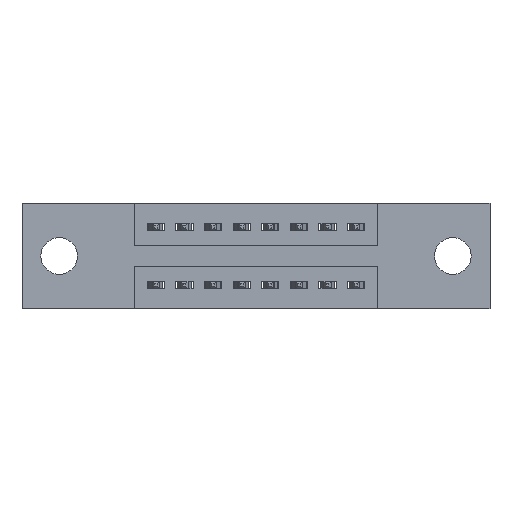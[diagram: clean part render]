
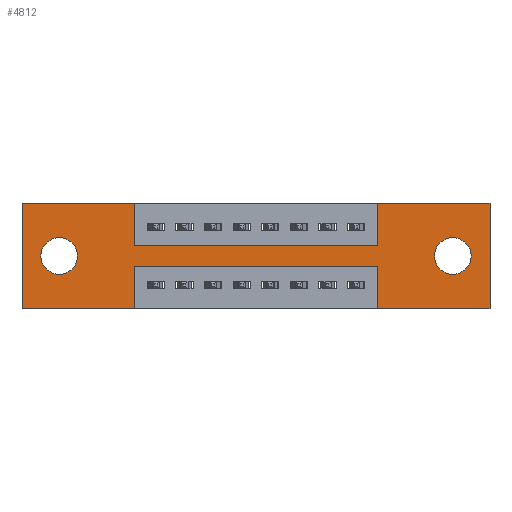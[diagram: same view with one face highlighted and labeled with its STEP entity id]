
A CAD part, front view. The second image highlights one B-rep face of the part: STEP entity #4812.
In plain terms, the highlighted planar face has unit normal (0, -1, 0).
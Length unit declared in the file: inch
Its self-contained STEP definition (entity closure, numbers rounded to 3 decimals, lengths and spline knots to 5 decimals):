
#135 = CARTESIAN_POINT ( 'NONE',  ( 0.13, 0., -0.121 ) ) ;
#247 = EDGE_CURVE ( 'NONE', #3289, #3170, #8852, .T. ) ;
#437 = LINE ( 'NONE', #5428, #8921 ) ;
#713 = VECTOR ( 'NONE', #811, 39.37008 ) ;
#737 = LINE ( 'NONE', #5722, #1028 ) ;
#811 = DIRECTION ( 'NONE',  ( 1., 0., 0. ) ) ;
#824 = CARTESIAN_POINT ( 'NONE',  ( 1.505, 0., -0.185 ) ) ;
#1003 = DIRECTION ( 'NONE',  ( 0., 0., -1. ) ) ;
#1018 = AXIS2_PLACEMENT_3D ( 'NONE', #5885, #7591, #2470 ) ;
#1028 = VECTOR ( 'NONE', #5741, 39.37008 ) ;
#1052 = LINE ( 'NONE', #7585, #7589 ) ;
#1186 = CARTESIAN_POINT ( 'NONE',  ( 1.2425, 0., -0.37 ) ) ;
#1396 = CARTESIAN_POINT ( 'NONE',  ( 0.3925, 0., -0.37 ) ) ;
#1403 = DIRECTION ( 'NONE',  ( 0., 0., 1. ) ) ;
#1425 = DIRECTION ( 'NONE',  ( 0., 1., 0. ) ) ;
#1453 = CARTESIAN_POINT ( 'NONE',  ( 0.13, 0., -0.185 ) ) ;
#1483 = VECTOR ( 'NONE', #7485, 39.37008 ) ;
#1489 = CARTESIAN_POINT ( 'NONE',  ( 0., 0., 0. ) ) ;
#1501 = LINE ( 'NONE', #4347, #5778 ) ;
#1685 = DIRECTION ( 'NONE',  ( 0., 0., -1. ) ) ;
#1695 = CARTESIAN_POINT ( 'NONE',  ( 1.2425, 0., -0.15 ) ) ;
#1724 = DIRECTION ( 'NONE',  ( 0., 0., 1. ) ) ;
#1790 = EDGE_CURVE ( 'NONE', #7550, #5250, #1052, .T. ) ;
#1797 = CARTESIAN_POINT ( 'NONE',  ( 1.635, 0., 0. ) ) ;
#1949 = CARTESIAN_POINT ( 'NONE',  ( 0.3925, 0., 0. ) ) ;
#1962 = CARTESIAN_POINT ( 'NONE',  ( 0.13, 0., -0.249 ) ) ;
#2136 = CARTESIAN_POINT ( 'NONE',  ( 0.3925, 0., -0.37 ) ) ;
#2155 = VERTEX_POINT ( 'NONE', #3154 ) ;
#2211 = CIRCLE ( 'NONE', #10122, 0.064 ) ;
#2331 = VECTOR ( 'NONE', #4119, 39.37008 ) ;
#2470 = DIRECTION ( 'NONE',  ( 0., 0., -1. ) ) ;
#2556 = ORIENTED_EDGE ( 'NONE', *, *, #7947, .T. ) ;
#2652 = VERTEX_POINT ( 'NONE', #7507 ) ;
#2775 = DIRECTION ( 'NONE',  ( 0., 1., 0. ) ) ;
#2778 = EDGE_CURVE ( 'NONE', #9200, #2155, #737, .T. ) ;
#2813 = ORIENTED_EDGE ( 'NONE', *, *, #3905, .T. ) ;
#2837 = EDGE_CURVE ( 'NONE', #2652, #10433, #437, .T. ) ;
#2843 = FACE_BOUND ( 'NONE', #8349, .T. ) ;
#2890 = CARTESIAN_POINT ( 'NONE',  ( 1.505, 0., -0.249 ) ) ;
#2953 = ORIENTED_EDGE ( 'NONE', *, *, #3360, .T. ) ;
#2977 = CARTESIAN_POINT ( 'NONE',  ( 0., 0., -0.37 ) ) ;
#3145 = ORIENTED_EDGE ( 'NONE', *, *, #5052, .T. ) ;
#3154 = CARTESIAN_POINT ( 'NONE',  ( 1.635, 0., -0.37 ) ) ;
#3158 = CIRCLE ( 'NONE', #6456, 0.064 ) ;
#3170 = VERTEX_POINT ( 'NONE', #2977 ) ;
#3173 = VERTEX_POINT ( 'NONE', #2890 ) ;
#3263 = DIRECTION ( 'NONE',  ( -1., 0., 0. ) ) ;
#3289 = VERTEX_POINT ( 'NONE', #2136 ) ;
#3360 = EDGE_CURVE ( 'NONE', #3510, #5759, #2211, .T. ) ;
#3379 = ORIENTED_EDGE ( 'NONE', *, *, #10715, .F. ) ;
#3394 = CARTESIAN_POINT ( 'NONE',  ( 1.2425, 0., 0. ) ) ;
#3510 = VERTEX_POINT ( 'NONE', #135 ) ;
#3530 = LINE ( 'NONE', #1489, #1483 ) ;
#3541 = DIRECTION ( 'NONE',  ( 0., 0., 1. ) ) ;
#3579 = CARTESIAN_POINT ( 'NONE',  ( 0.3925, 0., -0.22 ) ) ;
#3625 = ORIENTED_EDGE ( 'NONE', *, *, #2837, .F. ) ;
#3709 = VERTEX_POINT ( 'NONE', #5908 ) ;
#3717 = EDGE_CURVE ( 'NONE', #3709, #7550, #9409, .T. ) ;
#3744 = ORIENTED_EDGE ( 'NONE', *, *, #9153, .F. ) ;
#3876 = ORIENTED_EDGE ( 'NONE', *, *, #10476, .F. ) ;
#3905 = EDGE_CURVE ( 'NONE', #3173, #7233, #3158, .T. ) ;
#3952 = VERTEX_POINT ( 'NONE', #1186 ) ;
#3996 = ORIENTED_EDGE ( 'NONE', *, *, #2778, .F. ) ;
#4068 = VECTOR ( 'NONE', #4788, 39.37008 ) ;
#4119 = DIRECTION ( 'NONE',  ( 0., 0., 1. ) ) ;
#4135 = ORIENTED_EDGE ( 'NONE', *, *, #5413, .F. ) ;
#4184 = ORIENTED_EDGE ( 'NONE', *, *, #5606, .F. ) ;
#4314 = EDGE_LOOP ( 'NONE', ( #3379, #3625, #3744, #3876, #3996, #4135, #4184, #4341, #4401, #4580, #4757, #4849 ) ) ;
#4332 = CARTESIAN_POINT ( 'NONE',  ( 1.2425, 0., -0.37 ) ) ;
#4341 = ORIENTED_EDGE ( 'NONE', *, *, #10721, .F. ) ;
#4347 = CARTESIAN_POINT ( 'NONE',  ( 1.2425, 0., 0. ) ) ;
#4401 = ORIENTED_EDGE ( 'NONE', *, *, #1790, .F. ) ;
#4469 = VECTOR ( 'NONE', #5323, 39.37008 ) ;
#4538 = CARTESIAN_POINT ( 'NONE',  ( 1.505, 0., -0.185 ) ) ;
#4580 = ORIENTED_EDGE ( 'NONE', *, *, #3717, .F. ) ;
#4589 = LINE ( 'NONE', #10731, #2331 ) ;
#4757 = ORIENTED_EDGE ( 'NONE', *, *, #10211, .F. ) ;
#4788 = DIRECTION ( 'NONE',  ( 0., 0., -1. ) ) ;
#4812 = ADVANCED_FACE ( 'NONE', ( #2843, #9503, #5108 ), #8364, .T. ) ;
#4849 = ORIENTED_EDGE ( 'NONE', *, *, #247, .F. ) ;
#4966 = CIRCLE ( 'NONE', #6754, 0.064 ) ;
#5052 = EDGE_CURVE ( 'NONE', #5759, #3510, #4966, .T. ) ;
#5108 = FACE_OUTER_BOUND ( 'NONE', #4314, .T. ) ;
#5250 = VERTEX_POINT ( 'NONE', #6411 ) ;
#5323 = DIRECTION ( 'NONE',  ( -1., 0., 0. ) ) ;
#5400 = DIRECTION ( 'NONE',  ( 0., 0., -1. ) ) ;
#5413 = EDGE_CURVE ( 'NONE', #7954, #9200, #3530, .T. ) ;
#5428 = CARTESIAN_POINT ( 'NONE',  ( 0.3925, 0., -0.22 ) ) ;
#5592 = DIRECTION ( 'NONE',  ( -1., 0., 0. ) ) ;
#5606 = EDGE_CURVE ( 'NONE', #9108, #7954, #1501, .T. ) ;
#5693 = DIRECTION ( 'NONE',  ( 1., 0., 0. ) ) ;
#5722 = CARTESIAN_POINT ( 'NONE',  ( 1.635, 0., 0. ) ) ;
#5741 = DIRECTION ( 'NONE',  ( 0., 0., -1. ) ) ;
#5759 = VERTEX_POINT ( 'NONE', #1962 ) ;
#5778 = VECTOR ( 'NONE', #3541, 39.37008 ) ;
#5885 = CARTESIAN_POINT ( 'NONE',  ( 0., 0., -0.37 ) ) ;
#5908 = CARTESIAN_POINT ( 'NONE',  ( 0., 0., 0. ) ) ;
#6223 = LINE ( 'NONE', #10262, #4469 ) ;
#6411 = CARTESIAN_POINT ( 'NONE',  ( 0.3925, 0., -0.15 ) ) ;
#6456 = AXIS2_PLACEMENT_3D ( 'NONE', #4538, #10343, #5400 ) ;
#6754 = AXIS2_PLACEMENT_3D ( 'NONE', #7866, #2775, #8656 ) ;
#6832 = DIRECTION ( 'NONE',  ( 0., 1., 0. ) ) ;
#7059 = VECTOR ( 'NONE', #1724, 39.37008 ) ;
#7233 = VERTEX_POINT ( 'NONE', #9864 ) ;
#7392 = CARTESIAN_POINT ( 'NONE',  ( 0.3925, 0., -0.15 ) ) ;
#7485 = DIRECTION ( 'NONE',  ( 1., 0., 0. ) ) ;
#7507 = CARTESIAN_POINT ( 'NONE',  ( 1.2425, 0., -0.22 ) ) ;
#7529 = AXIS2_PLACEMENT_3D ( 'NONE', #824, #6832, #1685 ) ;
#7550 = VERTEX_POINT ( 'NONE', #1949 ) ;
#7585 = CARTESIAN_POINT ( 'NONE',  ( 0.3925, 0., 0. ) ) ;
#7589 = VECTOR ( 'NONE', #1003, 39.37008 ) ;
#7591 = DIRECTION ( 'NONE',  ( 0., -1., 0. ) ) ;
#7842 = CARTESIAN_POINT ( 'NONE',  ( 0., 0., -0.37 ) ) ;
#7848 = EDGE_LOOP ( 'NONE', ( #2953, #3145 ) ) ;
#7866 = CARTESIAN_POINT ( 'NONE',  ( 0.13, 0., -0.185 ) ) ;
#7947 = EDGE_CURVE ( 'NONE', #7233, #3173, #10608, .T. ) ;
#7954 = VERTEX_POINT ( 'NONE', #3394 ) ;
#8026 = VECTOR ( 'NONE', #5693, 39.37008 ) ;
#8349 = EDGE_LOOP ( 'NONE', ( #2556, #2813 ) ) ;
#8364 = PLANE ( 'NONE',  #1018 ) ;
#8656 = DIRECTION ( 'NONE',  ( 0., 0., 1. ) ) ;
#8852 = LINE ( 'NONE', #7842, #10508 ) ;
#8919 = LINE ( 'NONE', #4332, #7059 ) ;
#8921 = VECTOR ( 'NONE', #5592, 39.37008 ) ;
#9108 = VERTEX_POINT ( 'NONE', #1695 ) ;
#9153 = EDGE_CURVE ( 'NONE', #3952, #2652, #8919, .T. ) ;
#9200 = VERTEX_POINT ( 'NONE', #1797 ) ;
#9236 = CARTESIAN_POINT ( 'NONE',  ( 0., 0., 0. ) ) ;
#9409 = LINE ( 'NONE', #9236, #713 ) ;
#9503 = FACE_BOUND ( 'NONE', #7848, .T. ) ;
#9864 = CARTESIAN_POINT ( 'NONE',  ( 1.505, 0., -0.121 ) ) ;
#10122 = AXIS2_PLACEMENT_3D ( 'NONE', #1453, #1425, #1403 ) ;
#10148 = LINE ( 'NONE', #7392, #8026 ) ;
#10211 = EDGE_CURVE ( 'NONE', #3170, #3709, #4589, .T. ) ;
#10262 = CARTESIAN_POINT ( 'NONE',  ( 0., 0., -0.37 ) ) ;
#10343 = DIRECTION ( 'NONE',  ( 0., 1., 0. ) ) ;
#10420 = LINE ( 'NONE', #1396, #4068 ) ;
#10433 = VERTEX_POINT ( 'NONE', #3579 ) ;
#10476 = EDGE_CURVE ( 'NONE', #2155, #3952, #6223, .T. ) ;
#10508 = VECTOR ( 'NONE', #3263, 39.37008 ) ;
#10608 = CIRCLE ( 'NONE', #7529, 0.064 ) ;
#10715 = EDGE_CURVE ( 'NONE', #10433, #3289, #10420, .T. ) ;
#10721 = EDGE_CURVE ( 'NONE', #5250, #9108, #10148, .T. ) ;
#10731 = CARTESIAN_POINT ( 'NONE',  ( 0., 0., 0. ) ) ;
